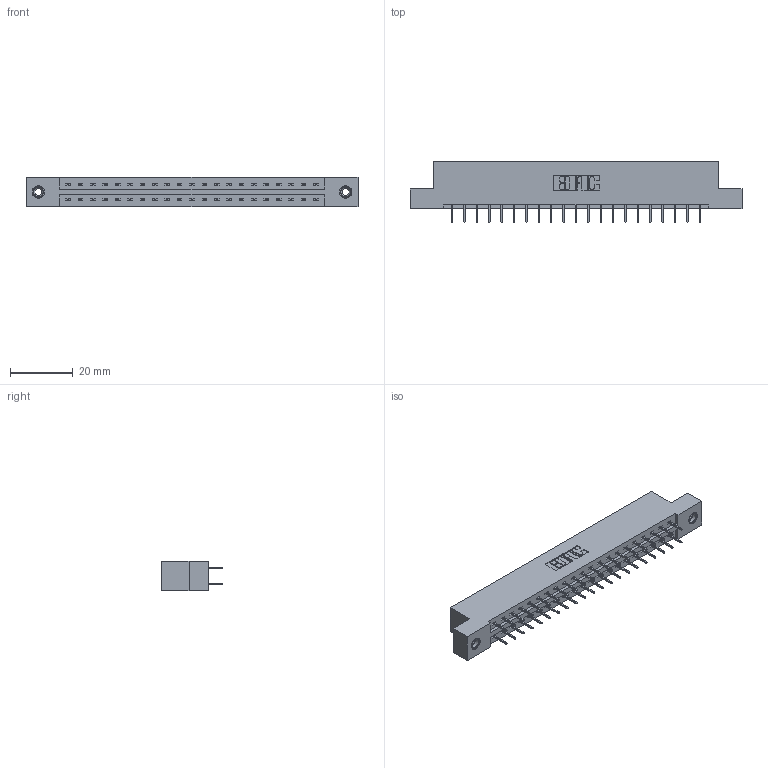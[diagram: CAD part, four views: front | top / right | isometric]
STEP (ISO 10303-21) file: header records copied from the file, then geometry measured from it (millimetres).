
FILE_DESCRIPTION (( 'STEP AP203' ), '1' );
FILE_NAME ('387-042-524-208.STEP', '2019-10-18T03:54:44', ( '' ), ( '' ), 'SwSTEP 2.0', 'SolidWorks 2016', '' );
FILE_SCHEMA (( 'CONFIG_CONTROL_DESIGN' ));
Length unit declared in the file: inch
Products named in the file (4): 337 Part_Flush Mounting Lugs - 0.156 Dia-TI; 345-292-001_345-293-124; 345-250-001_345-250-003-102; 387-042-524-208
Assembly tree (45 placements, depth 2):
  387-042-524-208
    337 Part_Flush Mounting Lugs - 0.156 Dia-TI
    345-292-001_345-293-124  x42
    345-250-001_345-250-003-102  x2
Bounding box: 106.22 x 19.69 x 9.4 mm (x, y, z)
Volume: 10845 mm3; surface area: 11883.4 mm2
Topology: 45 solids, 45 shells, 2610 faces, 7377 edges, 4742 vertices
Faces by surface type: plane 1950, cylinder 644, cone 12, torus 4
Entity records: 20258 total; most frequent: CARTESIAN_POINT 3409, ORIENTED_EDGE 3338, DIRECTION 2971, EDGE_CURVE 1669, LINE 1525, VECTOR 1525, VERTEX_POINT 1104, AXIS2_PLACEMENT_3D 723
